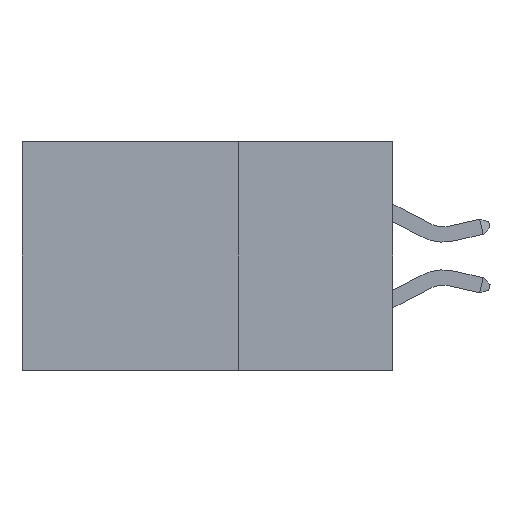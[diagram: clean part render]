
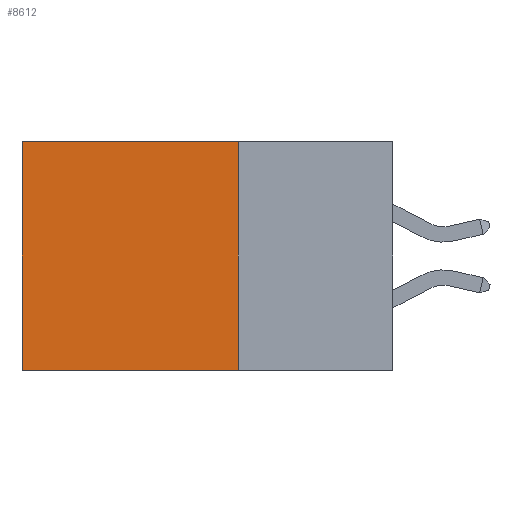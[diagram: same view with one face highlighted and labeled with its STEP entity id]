
A CAD part, left-side view. The second image highlights one B-rep face of the part: STEP entity #8612.
In plain terms, the highlighted planar face has unit normal (-1, 0, 0).
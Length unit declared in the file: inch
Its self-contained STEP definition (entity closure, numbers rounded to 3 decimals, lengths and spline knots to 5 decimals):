
#469 = LINE ( 'NONE', #16093, #7215 ) ;
#1123 = DIRECTION ( 'NONE',  ( 0., 0., -1. ) ) ;
#1336 = AXIS2_PLACEMENT_3D ( 'NONE', #5844, #20910, #1123 ) ;
#3702 = VERTEX_POINT ( 'NONE', #15543 ) ;
#3730 = DIRECTION ( 'NONE',  ( 0., 0., -1. ) ) ;
#4889 = EDGE_CURVE ( 'NONE', #13240, #5662, #27448, .T. ) ;
#5030 = ORIENTED_EDGE ( 'NONE', *, *, #11413, .T. ) ;
#5662 = VERTEX_POINT ( 'NONE', #14236 ) ;
#5844 = CARTESIAN_POINT ( 'NONE',  ( 0.2875, 0.25, 0. ) ) ;
#5974 = ORIENTED_EDGE ( 'NONE', *, *, #4889, .F. ) ;
#6578 = DIRECTION ( 'NONE',  ( 0., 0., -1. ) ) ;
#7215 = VECTOR ( 'NONE', #11823, 39.37008 ) ;
#8071 = CARTESIAN_POINT ( 'NONE',  ( 0.2875, 0.6, 0. ) ) ;
#8083 = FACE_OUTER_BOUND ( 'NONE', #18329, .T. ) ;
#8096 = CARTESIAN_POINT ( 'NONE',  ( 0.2875, 0.25, -0.37 ) ) ;
#8452 = ORIENTED_EDGE ( 'NONE', *, *, #26851, .T. ) ;
#8612 = ADVANCED_FACE ( 'NONE', ( #8083 ), #16269, .F. ) ;
#10599 = DIRECTION ( 'NONE',  ( 0., 1., 0. ) ) ;
#11117 = ORIENTED_EDGE ( 'NONE', *, *, #17902, .F. ) ;
#11413 = EDGE_CURVE ( 'NONE', #26811, #3702, #469, .T. ) ;
#11585 = VECTOR ( 'NONE', #10599, 39.37008 ) ;
#11823 = DIRECTION ( 'NONE',  ( 0., 1., 0. ) ) ;
#12923 = CARTESIAN_POINT ( 'NONE',  ( 0.2875, 0.25, 0. ) ) ;
#13240 = VERTEX_POINT ( 'NONE', #14291 ) ;
#14236 = CARTESIAN_POINT ( 'NONE',  ( 0.2875, 0.6, -0.37 ) ) ;
#14291 = CARTESIAN_POINT ( 'NONE',  ( 0.2875, 0.25, -0.37 ) ) ;
#14825 = VECTOR ( 'NONE', #3730, 39.37008 ) ;
#15148 = LINE ( 'NONE', #12923, #24569 ) ;
#15543 = CARTESIAN_POINT ( 'NONE',  ( 0.2875, 0.6, 0. ) ) ;
#16093 = CARTESIAN_POINT ( 'NONE',  ( 0.2875, 0.25, 0. ) ) ;
#16269 = PLANE ( 'NONE',  #1336 ) ;
#16510 = CARTESIAN_POINT ( 'NONE',  ( 0.2875, 0.25, 0. ) ) ;
#17902 = EDGE_CURVE ( 'NONE', #26811, #13240, #15148, .T. ) ;
#18329 = EDGE_LOOP ( 'NONE', ( #8452, #5974, #11117, #5030 ) ) ;
#20910 = DIRECTION ( 'NONE',  ( 1., 0., 0. ) ) ;
#22890 = LINE ( 'NONE', #8071, #14825 ) ;
#24569 = VECTOR ( 'NONE', #6578, 39.37008 ) ;
#26811 = VERTEX_POINT ( 'NONE', #16510 ) ;
#26851 = EDGE_CURVE ( 'NONE', #3702, #5662, #22890, .T. ) ;
#27448 = LINE ( 'NONE', #8096, #11585 ) ;
